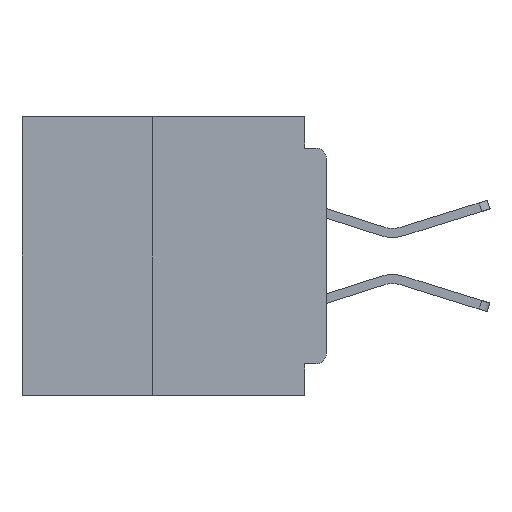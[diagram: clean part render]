
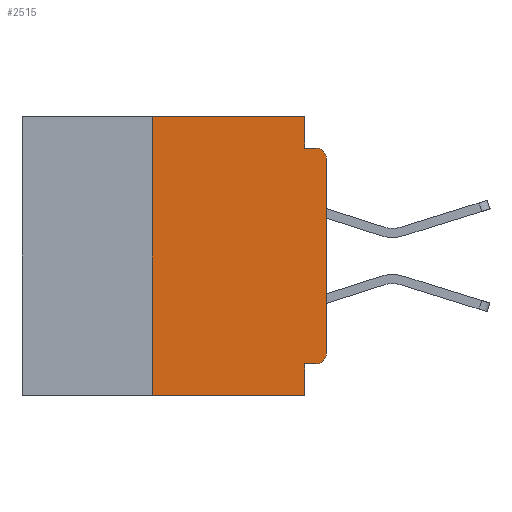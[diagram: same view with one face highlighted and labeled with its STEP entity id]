
A CAD part, left-side view. The second image highlights one B-rep face of the part: STEP entity #2515.
In plain terms, the highlighted planar face has unit normal (-1, 0, 0).
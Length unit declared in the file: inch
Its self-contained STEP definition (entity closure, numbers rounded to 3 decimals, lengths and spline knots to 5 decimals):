
#219 = LINE ( 'NONE', #17543, #59684 ) ;
#1727 = VERTEX_POINT ( 'NONE', #16437 ) ;
#1835 = CARTESIAN_POINT ( 'NONE',  ( 0., 0.015, -0.355 ) ) ;
#1938 = DIRECTION ( 'NONE',  ( -1., 0., 0. ) ) ;
#2515 = ADVANCED_FACE ( 'NONE', ( #24715 ), #54738, .F. ) ;
#2765 = AXIS2_PLACEMENT_3D ( 'NONE', #30297, #1938, #35027 ) ;
#2824 = LINE ( 'NONE', #21328, #39025 ) ;
#2991 = CARTESIAN_POINT ( 'NONE',  ( 0., 0., -0.045 ) ) ;
#4841 = VECTOR ( 'NONE', #13430, 39.37008 ) ;
#6032 = CARTESIAN_POINT ( 'NONE',  ( 0., 0., -0.34 ) ) ;
#6691 = VECTOR ( 'NONE', #57276, 39.37008 ) ;
#7657 = LINE ( 'NONE', #17835, #18746 ) ;
#7658 = VECTOR ( 'NONE', #26496, 39.37008 ) ;
#8173 = ORIENTED_EDGE ( 'NONE', *, *, #41035, .F. ) ;
#8692 = CARTESIAN_POINT ( 'NONE',  ( 0., 0.25, -0.4 ) ) ;
#9384 = VERTEX_POINT ( 'NONE', #6032 ) ;
#11127 = LINE ( 'NONE', #28113, #22226 ) ;
#11587 = VERTEX_POINT ( 'NONE', #52483 ) ;
#12218 = AXIS2_PLACEMENT_3D ( 'NONE', #12573, #26830, #59389 ) ;
#12221 = VERTEX_POINT ( 'NONE', #47527 ) ;
#12573 = CARTESIAN_POINT ( 'NONE',  ( 0., 0.437, 0. ) ) ;
#13430 = DIRECTION ( 'NONE',  ( 0., 0., 1. ) ) ;
#13795 = VECTOR ( 'NONE', #26604, 39.37008 ) ;
#14205 = ORIENTED_EDGE ( 'NONE', *, *, #16163, .F. ) ;
#14277 = VERTEX_POINT ( 'NONE', #58956 ) ;
#15266 = LINE ( 'NONE', #2991, #13795 ) ;
#15387 = LINE ( 'NONE', #35965, #7658 ) ;
#15535 = ORIENTED_EDGE ( 'NONE', *, *, #24359, .T. ) ;
#16163 = EDGE_CURVE ( 'NONE', #11587, #52391, #15266, .T. ) ;
#16266 = ORIENTED_EDGE ( 'NONE', *, *, #39172, .T. ) ;
#16437 = CARTESIAN_POINT ( 'NONE',  ( 0., 0.25, -0.4 ) ) ;
#17019 = AXIS2_PLACEMENT_3D ( 'NONE', #56004, #28115, #60657 ) ;
#17543 = CARTESIAN_POINT ( 'NONE',  ( 0., 0., 0. ) ) ;
#17835 = CARTESIAN_POINT ( 'NONE',  ( 0., 0., -0.355 ) ) ;
#18625 = DIRECTION ( 'NONE',  ( 0., 0., -1. ) ) ;
#18644 = ORIENTED_EDGE ( 'NONE', *, *, #37681, .T. ) ;
#18741 = CARTESIAN_POINT ( 'NONE',  ( 0., 0.031, -0.4 ) ) ;
#18746 = VECTOR ( 'NONE', #55229, 39.37008 ) ;
#19849 = EDGE_CURVE ( 'NONE', #1727, #47868, #42461, .T. ) ;
#21328 = CARTESIAN_POINT ( 'NONE',  ( 0., 0.031, -0.4 ) ) ;
#22226 = VECTOR ( 'NONE', #18625, 39.37008 ) ;
#24359 = EDGE_CURVE ( 'NONE', #1727, #33894, #15387, .T. ) ;
#24554 = EDGE_CURVE ( 'NONE', #51763, #9384, #48264, .T. ) ;
#24695 = CARTESIAN_POINT ( 'NONE',  ( 0., 0.437, 0. ) ) ;
#24715 = FACE_OUTER_BOUND ( 'NONE', #34241, .T. ) ;
#26496 = DIRECTION ( 'NONE',  ( 0., -1., 0. ) ) ;
#26604 = DIRECTION ( 'NONE',  ( 0., -1., 0. ) ) ;
#26830 = DIRECTION ( 'NONE',  ( 1., 0., 0. ) ) ;
#28113 = CARTESIAN_POINT ( 'NONE',  ( 0., 0.031, 0. ) ) ;
#28115 = DIRECTION ( 'NONE',  ( -1., 0., 0. ) ) ;
#29922 = CARTESIAN_POINT ( 'NONE',  ( 0., 0.015, -0.045 ) ) ;
#30297 = CARTESIAN_POINT ( 'NONE',  ( 0., 0.015, -0.06 ) ) ;
#32727 = ORIENTED_EDGE ( 'NONE', *, *, #19849, .F. ) ;
#32990 = CIRCLE ( 'NONE', #2765, 0.015 ) ;
#33788 = ORIENTED_EDGE ( 'NONE', *, *, #51112, .F. ) ;
#33894 = VERTEX_POINT ( 'NONE', #18741 ) ;
#34241 = EDGE_LOOP ( 'NONE', ( #16266, #18644, #14205, #33788, #8173, #32727, #15535, #51775, #37356, #58309 ) ) ;
#34888 = EDGE_CURVE ( 'NONE', #51763, #14277, #7657, .T. ) ;
#35027 = DIRECTION ( 'NONE',  ( 0., 0., -1. ) ) ;
#35150 = CARTESIAN_POINT ( 'NONE',  ( 0., 0.25, 0. ) ) ;
#35965 = CARTESIAN_POINT ( 'NONE',  ( 0., 0.437, -0.4 ) ) ;
#36289 = DIRECTION ( 'NONE',  ( 0., 0., 1. ) ) ;
#37356 = ORIENTED_EDGE ( 'NONE', *, *, #34888, .F. ) ;
#37681 = EDGE_CURVE ( 'NONE', #12221, #52391, #32990, .T. ) ;
#39025 = VECTOR ( 'NONE', #44828, 39.37008 ) ;
#39172 = EDGE_CURVE ( 'NONE', #9384, #12221, #219, .T. ) ;
#41035 = EDGE_CURVE ( 'NONE', #47868, #56211, #55087, .T. ) ;
#42461 = LINE ( 'NONE', #8692, #4841 ) ;
#44828 = DIRECTION ( 'NONE',  ( 0., 0., -1. ) ) ;
#46881 = CARTESIAN_POINT ( 'NONE',  ( 0., 0.031, 0. ) ) ;
#47527 = CARTESIAN_POINT ( 'NONE',  ( 0., 0., -0.06 ) ) ;
#47868 = VERTEX_POINT ( 'NONE', #35150 ) ;
#48264 = CIRCLE ( 'NONE', #17019, 0.015 ) ;
#51112 = EDGE_CURVE ( 'NONE', #56211, #11587, #11127, .T. ) ;
#51763 = VERTEX_POINT ( 'NONE', #1835 ) ;
#51775 = ORIENTED_EDGE ( 'NONE', *, *, #51875, .F. ) ;
#51875 = EDGE_CURVE ( 'NONE', #14277, #33894, #2824, .T. ) ;
#52391 = VERTEX_POINT ( 'NONE', #29922 ) ;
#52483 = CARTESIAN_POINT ( 'NONE',  ( 0., 0.031, -0.045 ) ) ;
#54738 = PLANE ( 'NONE',  #12218 ) ;
#55087 = LINE ( 'NONE', #24695, #6691 ) ;
#55229 = DIRECTION ( 'NONE',  ( 0., 1., 0. ) ) ;
#56004 = CARTESIAN_POINT ( 'NONE',  ( 0., 0.015, -0.34 ) ) ;
#56211 = VERTEX_POINT ( 'NONE', #46881 ) ;
#57276 = DIRECTION ( 'NONE',  ( 0., -1., 0. ) ) ;
#58309 = ORIENTED_EDGE ( 'NONE', *, *, #24554, .T. ) ;
#58956 = CARTESIAN_POINT ( 'NONE',  ( 0., 0.031, -0.355 ) ) ;
#59389 = DIRECTION ( 'NONE',  ( 0., 0., -1. ) ) ;
#59684 = VECTOR ( 'NONE', #36289, 39.37008 ) ;
#60657 = DIRECTION ( 'NONE',  ( 0., 0., -1. ) ) ;
